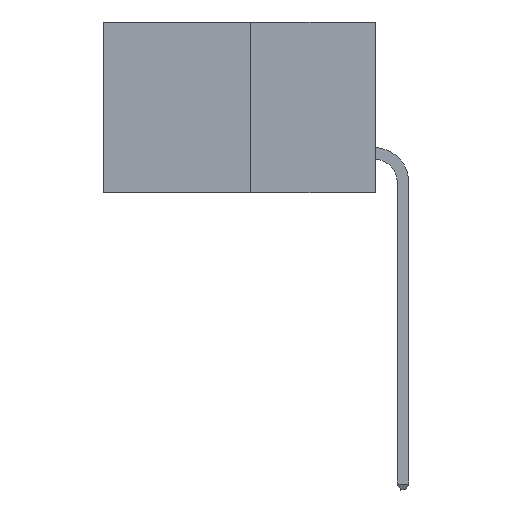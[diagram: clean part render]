
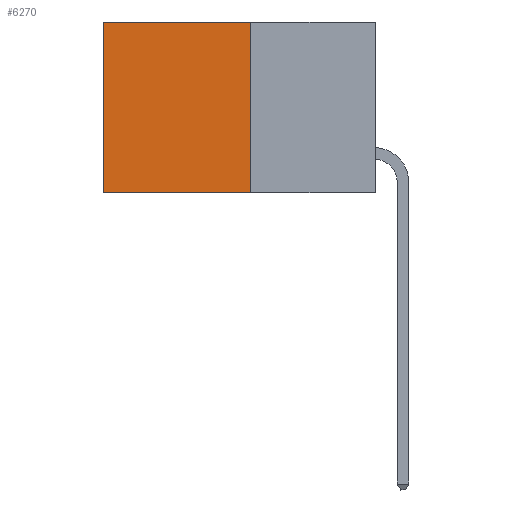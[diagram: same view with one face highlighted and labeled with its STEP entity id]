
A CAD part, left-side view. The second image highlights one B-rep face of the part: STEP entity #6270.
In plain terms, the highlighted planar face has unit normal (-1, 0, 0).
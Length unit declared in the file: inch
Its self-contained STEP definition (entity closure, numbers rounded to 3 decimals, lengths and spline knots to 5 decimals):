
#3 = LINE ( 'NONE', #2732, #12200 ) ;
#158 = VECTOR ( 'NONE', #12504, 39.37008 ) ;
#612 = DIRECTION ( 'NONE',  ( 0., 1., 0. ) ) ;
#639 = CARTESIAN_POINT ( 'NONE',  ( 0.277, 0.27, -0.37 ) ) ;
#1084 = CARTESIAN_POINT ( 'NONE',  ( 0.277, 0.59, -0.37 ) ) ;
#1450 = LINE ( 'NONE', #7857, #7283 ) ;
#1584 = ORIENTED_EDGE ( 'NONE', *, *, #5195, .F. ) ;
#2010 = EDGE_CURVE ( 'NONE', #11681, #5500, #5083, .T. ) ;
#2492 = AXIS2_PLACEMENT_3D ( 'NONE', #10253, #11325, #4846 ) ;
#2732 = CARTESIAN_POINT ( 'NONE',  ( 0.277, 0.27, -0.37 ) ) ;
#3540 = LINE ( 'NONE', #11432, #158 ) ;
#3670 = CARTESIAN_POINT ( 'NONE',  ( 0.277, 0.59, 0. ) ) ;
#3818 = EDGE_CURVE ( 'NONE', #4228, #5559, #1450, .T. ) ;
#4228 = VERTEX_POINT ( 'NONE', #5601 ) ;
#4798 = CARTESIAN_POINT ( 'NONE',  ( 0.277, 0.27, -0.37 ) ) ;
#4846 = DIRECTION ( 'NONE',  ( 0., 0., -1. ) ) ;
#5083 = LINE ( 'NONE', #639, #10493 ) ;
#5195 = EDGE_CURVE ( 'NONE', #4228, #11681, #3, .T. ) ;
#5500 = VERTEX_POINT ( 'NONE', #1084 ) ;
#5559 = VERTEX_POINT ( 'NONE', #3670 ) ;
#5601 = CARTESIAN_POINT ( 'NONE',  ( 0.277, 0.27, 0. ) ) ;
#6270 = ADVANCED_FACE ( 'NONE', ( #11995 ), #8136, .F. ) ;
#7283 = VECTOR ( 'NONE', #7740, 39.37008 ) ;
#7740 = DIRECTION ( 'NONE',  ( 0., 1., 0. ) ) ;
#7857 = CARTESIAN_POINT ( 'NONE',  ( 0.277, 0.27, 0. ) ) ;
#8136 = PLANE ( 'NONE',  #2492 ) ;
#8931 = EDGE_LOOP ( 'NONE', ( #10125, #10249, #1584, #9308 ) ) ;
#9308 = ORIENTED_EDGE ( 'NONE', *, *, #3818, .T. ) ;
#10125 = ORIENTED_EDGE ( 'NONE', *, *, #10968, .T. ) ;
#10249 = ORIENTED_EDGE ( 'NONE', *, *, #2010, .F. ) ;
#10253 = CARTESIAN_POINT ( 'NONE',  ( 0.277, 0.27, -0.37 ) ) ;
#10493 = VECTOR ( 'NONE', #612, 39.37008 ) ;
#10522 = DIRECTION ( 'NONE',  ( 0., 0., -1. ) ) ;
#10968 = EDGE_CURVE ( 'NONE', #5559, #5500, #3540, .T. ) ;
#11325 = DIRECTION ( 'NONE',  ( 1., 0., 0. ) ) ;
#11432 = CARTESIAN_POINT ( 'NONE',  ( 0.277, 0.59, -0.37 ) ) ;
#11681 = VERTEX_POINT ( 'NONE', #4798 ) ;
#11995 = FACE_OUTER_BOUND ( 'NONE', #8931, .T. ) ;
#12200 = VECTOR ( 'NONE', #10522, 39.37008 ) ;
#12504 = DIRECTION ( 'NONE',  ( 0., 0., -1. ) ) ;
